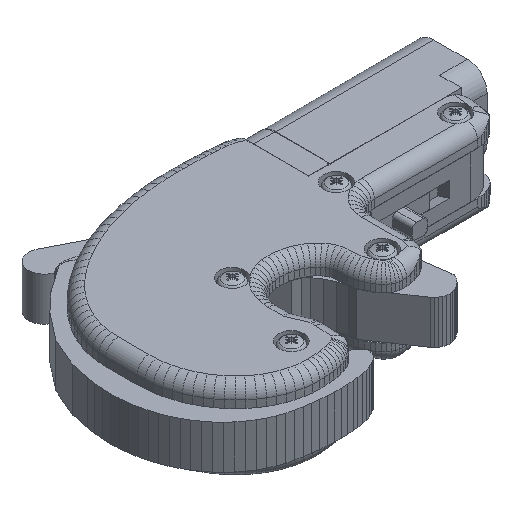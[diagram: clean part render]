
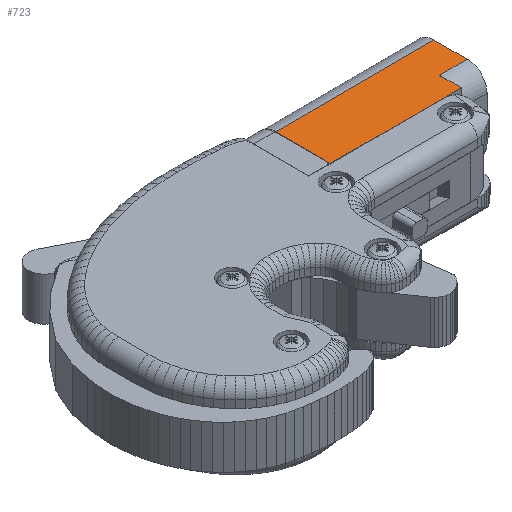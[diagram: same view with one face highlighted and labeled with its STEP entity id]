
A CAD part, isometric view. The second image highlights one B-rep face of the part: STEP entity #723.
In plain terms, the highlighted planar face has unit normal (0, 0, 1).
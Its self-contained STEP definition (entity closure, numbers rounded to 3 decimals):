
#282=CARTESIAN_POINT('',(13.31,10.229,16.0));
#283=VERTEX_POINT('',#282);
#291=CARTESIAN_POINT('',(6.287,10.229,16.));
#292=VERTEX_POINT('',#291);
#293=CARTESIAN_POINT('',(13.31,10.229,16.));
#294=DIRECTION('',(-1.0,0.0,0.0));
#295=VECTOR('',#294,7.023);
#296=LINE('',#293,#295);
#297=EDGE_CURVE('',#283,#292,#296,.T.);
#365=CARTESIAN_POINT('',(13.31,18.729,16.0));
#366=VERTEX_POINT('',#365);
#374=CARTESIAN_POINT('',(13.31,18.729,16.0));
#375=DIRECTION('',(0.0,-1.0,0.0));
#376=VECTOR('',#375,8.5);
#377=LINE('',#374,#376);
#378=EDGE_CURVE('',#366,#283,#377,.T.);
#490=CARTESIAN_POINT('',(6.287,4.729,16.0));
#491=VERTEX_POINT('',#490);
#516=CARTESIAN_POINT('',(6.287,4.729,16.));
#517=DIRECTION('',(0.0,1.0,0.0));
#518=VECTOR('',#517,5.5);
#519=LINE('',#516,#518);
#520=EDGE_CURVE('',#491,#292,#519,.T.);
#614=CARTESIAN_POINT('',(-27.006,18.729,16.0));
#615=VERTEX_POINT('',#614);
#623=CARTESIAN_POINT('',(-27.006,18.729,16.));
#624=DIRECTION('',(1.0,0.0,0.0));
#625=VECTOR('',#624,40.316);
#626=LINE('',#623,#625);
#627=EDGE_CURVE('',#615,#366,#626,.T.);
#680=CARTESIAN_POINT('',(-27.006,4.729,16.0));
#681=VERTEX_POINT('',#680);
#682=CARTESIAN_POINT('',(-27.006,4.729,16.0));
#683=DIRECTION('',(1.0,0.0,0.0));
#684=VECTOR('',#683,33.293);
#685=LINE('',#682,#684);
#686=EDGE_CURVE('',#681,#491,#685,.T.);
#705=CARTESIAN_POINT('',(-10.348,14.229,16.));
#706=DIRECTION('',(0.0,0.0,1.0));
#707=DIRECTION('',(1.0,0.0,0.0));
#708=AXIS2_PLACEMENT_3D('',#705,#706,#707);
#709=PLANE('',#708);
#710=ORIENTED_EDGE('',*,*,#297,.F.);
#711=ORIENTED_EDGE('',*,*,#378,.F.);
#712=ORIENTED_EDGE('',*,*,#627,.F.);
#713=CARTESIAN_POINT('',(-27.006,18.729,16.0));
#714=DIRECTION('',(0.0,-1.0,0.0));
#715=VECTOR('',#714,14.0);
#716=LINE('',#713,#715);
#717=EDGE_CURVE('',#615,#681,#716,.T.);
#718=ORIENTED_EDGE('',*,*,#717,.T.);
#719=ORIENTED_EDGE('',*,*,#686,.T.);
#720=ORIENTED_EDGE('',*,*,#520,.T.);
#721=EDGE_LOOP('',(#710,#711,#712,#718,#719,#720));
#722=FACE_OUTER_BOUND('',#721,.T.);
#723=ADVANCED_FACE('',(#722),#709,.T.);
